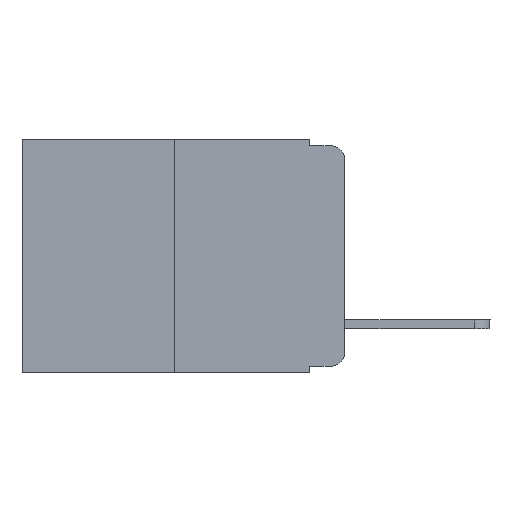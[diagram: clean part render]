
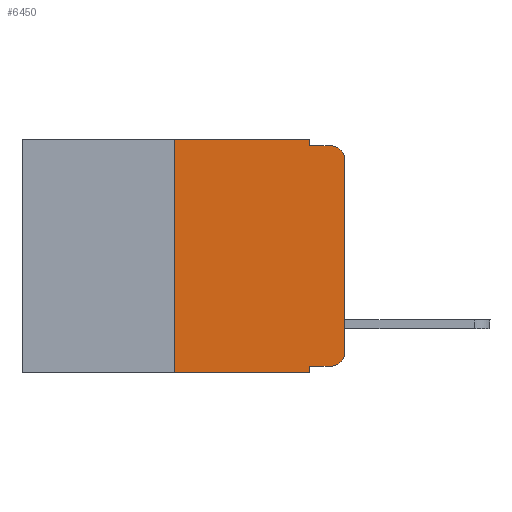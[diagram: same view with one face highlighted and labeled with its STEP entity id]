
A CAD part, left-side view. The second image highlights one B-rep face of the part: STEP entity #6450.
In plain terms, the highlighted planar face has unit normal (-1, 0, 0).
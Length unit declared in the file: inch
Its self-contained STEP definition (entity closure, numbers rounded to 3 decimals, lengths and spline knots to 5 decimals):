
#187 = EDGE_CURVE ( 'NONE', #9203, #9776, #5871, .T. ) ;
#284 = CARTESIAN_POINT ( 'NONE',  ( 0., 0., -0.313 ) ) ;
#406 = AXIS2_PLACEMENT_3D ( 'NONE', #9970, #5063, #5906 ) ;
#591 = CARTESIAN_POINT ( 'NONE',  ( 0., 0.051, 0. ) ) ;
#635 = VERTEX_POINT ( 'NONE', #4549 ) ;
#656 = CARTESIAN_POINT ( 'NONE',  ( 0., 0.25, 0. ) ) ;
#696 = DIRECTION ( 'NONE',  ( 0., -1., 0. ) ) ;
#1233 = CARTESIAN_POINT ( 'NONE',  ( 0., 0.051, -0.01 ) ) ;
#1530 = ORIENTED_EDGE ( 'NONE', *, *, #10380, .F. ) ;
#1747 = ORIENTED_EDGE ( 'NONE', *, *, #4838, .T. ) ;
#2221 = AXIS2_PLACEMENT_3D ( 'NONE', #6789, #8792, #2834 ) ;
#2262 = AXIS2_PLACEMENT_3D ( 'NONE', #10503, #4527, #11490 ) ;
#2824 = CARTESIAN_POINT ( 'NONE',  ( 0., 0.02, -0.333 ) ) ;
#2834 = DIRECTION ( 'NONE',  ( 0., 0., -1. ) ) ;
#2856 = VECTOR ( 'NONE', #9940, 39.37008 ) ;
#2935 = CARTESIAN_POINT ( 'NONE',  ( 0., 0., 0. ) ) ;
#3392 = CARTESIAN_POINT ( 'NONE',  ( 0., 0.02, -0.01 ) ) ;
#3455 = ORIENTED_EDGE ( 'NONE', *, *, #12704, .T. ) ;
#3530 = VECTOR ( 'NONE', #6879, 39.37008 ) ;
#3657 = VECTOR ( 'NONE', #9783, 39.37008 ) ;
#3784 = LINE ( 'NONE', #2935, #2856 ) ;
#3919 = VECTOR ( 'NONE', #8132, 39.37008 ) ;
#4288 = LINE ( 'NONE', #656, #12729 ) ;
#4519 = FACE_OUTER_BOUND ( 'NONE', #4565, .T. ) ;
#4527 = DIRECTION ( 'NONE',  ( 1., 0., 0. ) ) ;
#4549 = CARTESIAN_POINT ( 'NONE',  ( 0., 0., -0.03 ) ) ;
#4565 = EDGE_LOOP ( 'NONE', ( #9188, #1747, #7565, #5708, #1530, #6419, #8930, #5727, #5258, #3455 ) ) ;
#4609 = PLANE ( 'NONE',  #2262 ) ;
#4641 = CARTESIAN_POINT ( 'NONE',  ( 0., 0.051, -0.333 ) ) ;
#4838 = EDGE_CURVE ( 'NONE', #635, #7054, #7167, .T. ) ;
#5063 = DIRECTION ( 'NONE',  ( -1., 0., 0. ) ) ;
#5258 = ORIENTED_EDGE ( 'NONE', *, *, #10208, .T. ) ;
#5316 = CARTESIAN_POINT ( 'NONE',  ( 0., 0.051, 0. ) ) ;
#5708 = ORIENTED_EDGE ( 'NONE', *, *, #8601, .F. ) ;
#5727 = ORIENTED_EDGE ( 'NONE', *, *, #187, .F. ) ;
#5871 = LINE ( 'NONE', #5316, #12928 ) ;
#5906 = DIRECTION ( 'NONE',  ( 0., 0., -1. ) ) ;
#6243 = LINE ( 'NONE', #1233, #3919 ) ;
#6279 = DIRECTION ( 'NONE',  ( 0., 0., -1. ) ) ;
#6412 = CARTESIAN_POINT ( 'NONE',  ( 0., 0.473, -0.343 ) ) ;
#6419 = ORIENTED_EDGE ( 'NONE', *, *, #10165, .F. ) ;
#6450 = ADVANCED_FACE ( 'NONE', ( #4519 ), #4609, .F. ) ;
#6648 = LINE ( 'NONE', #12875, #3530 ) ;
#6701 = DIRECTION ( 'NONE',  ( 0., 0., 1. ) ) ;
#6789 = CARTESIAN_POINT ( 'NONE',  ( 0., 0.02, -0.313 ) ) ;
#6879 = DIRECTION ( 'NONE',  ( 0., 0., -1. ) ) ;
#7054 = VERTEX_POINT ( 'NONE', #3392 ) ;
#7167 = CIRCLE ( 'NONE', #406, 0.02 ) ;
#7565 = ORIENTED_EDGE ( 'NONE', *, *, #12276, .F. ) ;
#7862 = VERTEX_POINT ( 'NONE', #12943 ) ;
#8003 = CARTESIAN_POINT ( 'NONE',  ( 0., 0.051, -0.343 ) ) ;
#8132 = DIRECTION ( 'NONE',  ( 0., -1., 0. ) ) ;
#8509 = VERTEX_POINT ( 'NONE', #12738 ) ;
#8521 = VECTOR ( 'NONE', #10280, 39.37008 ) ;
#8601 = EDGE_CURVE ( 'NONE', #11793, #10071, #6648, .T. ) ;
#8792 = DIRECTION ( 'NONE',  ( -1., 0., 0. ) ) ;
#8920 = CARTESIAN_POINT ( 'NONE',  ( 0., 0.473, 0. ) ) ;
#8930 = ORIENTED_EDGE ( 'NONE', *, *, #9416, .T. ) ;
#9188 = ORIENTED_EDGE ( 'NONE', *, *, #11596, .T. ) ;
#9203 = VERTEX_POINT ( 'NONE', #10034 ) ;
#9335 = VERTEX_POINT ( 'NONE', #284 ) ;
#9416 = EDGE_CURVE ( 'NONE', #8509, #9776, #10999, .T. ) ;
#9572 = VECTOR ( 'NONE', #696, 39.37008 ) ;
#9776 = VERTEX_POINT ( 'NONE', #8003 ) ;
#9783 = DIRECTION ( 'NONE',  ( 0., -1., 0. ) ) ;
#9940 = DIRECTION ( 'NONE',  ( 0., 0., 1. ) ) ;
#9970 = CARTESIAN_POINT ( 'NONE',  ( 0., 0.02, -0.03 ) ) ;
#10034 = CARTESIAN_POINT ( 'NONE',  ( 0., 0.051, -0.333 ) ) ;
#10046 = LINE ( 'NONE', #8920, #3657 ) ;
#10071 = VERTEX_POINT ( 'NONE', #12454 ) ;
#10165 = EDGE_CURVE ( 'NONE', #8509, #7862, #4288, .T. ) ;
#10208 = EDGE_CURVE ( 'NONE', #9203, #10730, #12717, .T. ) ;
#10280 = DIRECTION ( 'NONE',  ( 0., -1., 0. ) ) ;
#10380 = EDGE_CURVE ( 'NONE', #7862, #11793, #10046, .T. ) ;
#10503 = CARTESIAN_POINT ( 'NONE',  ( 0., 0.473, 0. ) ) ;
#10730 = VERTEX_POINT ( 'NONE', #2824 ) ;
#10999 = LINE ( 'NONE', #6412, #8521 ) ;
#11490 = DIRECTION ( 'NONE',  ( 0., 0., -1. ) ) ;
#11596 = EDGE_CURVE ( 'NONE', #9335, #635, #3784, .T. ) ;
#11793 = VERTEX_POINT ( 'NONE', #591 ) ;
#12276 = EDGE_CURVE ( 'NONE', #10071, #7054, #6243, .T. ) ;
#12454 = CARTESIAN_POINT ( 'NONE',  ( 0., 0.051, -0.01 ) ) ;
#12704 = EDGE_CURVE ( 'NONE', #10730, #9335, #12906, .T. ) ;
#12717 = LINE ( 'NONE', #4641, #9572 ) ;
#12729 = VECTOR ( 'NONE', #6701, 39.37008 ) ;
#12738 = CARTESIAN_POINT ( 'NONE',  ( 0., 0.25, -0.343 ) ) ;
#12875 = CARTESIAN_POINT ( 'NONE',  ( 0., 0.051, 0. ) ) ;
#12906 = CIRCLE ( 'NONE', #2221, 0.02 ) ;
#12928 = VECTOR ( 'NONE', #6279, 39.37008 ) ;
#12943 = CARTESIAN_POINT ( 'NONE',  ( 0., 0.25, 0. ) ) ;
